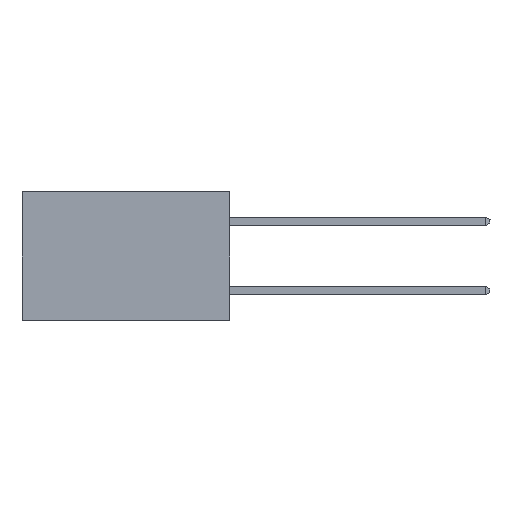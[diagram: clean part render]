
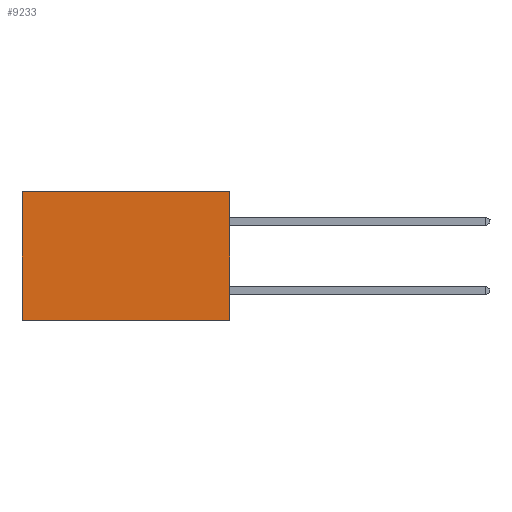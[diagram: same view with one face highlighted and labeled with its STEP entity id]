
A CAD part, left-side view. The second image highlights one B-rep face of the part: STEP entity #9233.
In plain terms, the highlighted planar face has unit normal (-1, 0, 0).
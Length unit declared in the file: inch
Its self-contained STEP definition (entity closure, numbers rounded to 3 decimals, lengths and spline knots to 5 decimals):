
#179 = LINE ( 'NONE', #12154, #4477 ) ;
#184 = ORIENTED_EDGE ( 'NONE', *, *, #5559, .F. ) ;
#1104 = DIRECTION ( 'NONE',  ( 1., 0., 0. ) ) ;
#1189 = AXIS2_PLACEMENT_3D ( 'NONE', #6382, #1104, #12731 ) ;
#1465 = VERTEX_POINT ( 'NONE', #12249 ) ;
#1660 = VERTEX_POINT ( 'NONE', #16393 ) ;
#3008 = CARTESIAN_POINT ( 'NONE',  ( 0.2615, 0.6, -0.37 ) ) ;
#3230 = EDGE_LOOP ( 'NONE', ( #6766, #184, #13836, #15476 ) ) ;
#4416 = EDGE_CURVE ( 'NONE', #1660, #11611, #11552, .T. ) ;
#4431 = DIRECTION ( 'NONE',  ( 0., 1., 0. ) ) ;
#4477 = VECTOR ( 'NONE', #4431, 39.37008 ) ;
#4557 = DIRECTION ( 'NONE',  ( 0., 1., 0. ) ) ;
#5004 = DIRECTION ( 'NONE',  ( 0., 0., -1. ) ) ;
#5559 = EDGE_CURVE ( 'NONE', #1465, #11611, #179, .T. ) ;
#5691 = CARTESIAN_POINT ( 'NONE',  ( 0.2615, 0., 0. ) ) ;
#6382 = CARTESIAN_POINT ( 'NONE',  ( 0.2615, 0., -0.37 ) ) ;
#6766 = ORIENTED_EDGE ( 'NONE', *, *, #4416, .T. ) ;
#7806 = VECTOR ( 'NONE', #4557, 39.37008 ) ;
#8544 = EDGE_CURVE ( 'NONE', #16756, #1660, #8628, .T. ) ;
#8628 = LINE ( 'NONE', #5691, #7806 ) ;
#8705 = DIRECTION ( 'NONE',  ( 0., 0., -1. ) ) ;
#9233 = ADVANCED_FACE ( 'NONE', ( #16698 ), #10088, .F. ) ;
#9982 = CARTESIAN_POINT ( 'NONE',  ( 0.2615, 0., -0.37 ) ) ;
#10088 = PLANE ( 'NONE',  #1189 ) ;
#10738 = CARTESIAN_POINT ( 'NONE',  ( 0.2615, 0.6, -0.37 ) ) ;
#11552 = LINE ( 'NONE', #10738, #13791 ) ;
#11611 = VERTEX_POINT ( 'NONE', #3008 ) ;
#12154 = CARTESIAN_POINT ( 'NONE',  ( 0.2615, 0., -0.37 ) ) ;
#12249 = CARTESIAN_POINT ( 'NONE',  ( 0.2615, 0., -0.37 ) ) ;
#12535 = LINE ( 'NONE', #9982, #14728 ) ;
#12731 = DIRECTION ( 'NONE',  ( 0., 0., -1. ) ) ;
#13791 = VECTOR ( 'NONE', #5004, 39.37008 ) ;
#13836 = ORIENTED_EDGE ( 'NONE', *, *, #14169, .F. ) ;
#14169 = EDGE_CURVE ( 'NONE', #16756, #1465, #12535, .T. ) ;
#14728 = VECTOR ( 'NONE', #8705, 39.37008 ) ;
#14885 = CARTESIAN_POINT ( 'NONE',  ( 0.2615, 0., 0. ) ) ;
#15476 = ORIENTED_EDGE ( 'NONE', *, *, #8544, .T. ) ;
#16393 = CARTESIAN_POINT ( 'NONE',  ( 0.2615, 0.6, 0. ) ) ;
#16698 = FACE_OUTER_BOUND ( 'NONE', #3230, .T. ) ;
#16756 = VERTEX_POINT ( 'NONE', #14885 ) ;
